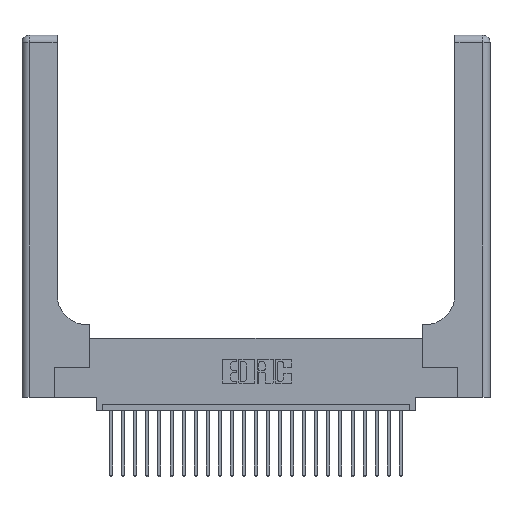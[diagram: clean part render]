
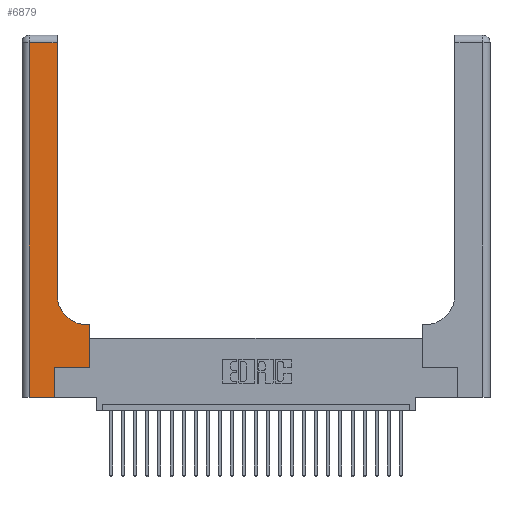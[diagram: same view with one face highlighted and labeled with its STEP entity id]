
A CAD part, top view. The second image highlights one B-rep face of the part: STEP entity #6879.
In plain terms, the highlighted planar face has unit normal (0, 0, 1).
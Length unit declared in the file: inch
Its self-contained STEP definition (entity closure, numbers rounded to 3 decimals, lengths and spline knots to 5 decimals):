
#257 = CARTESIAN_POINT ( 'NONE',  ( 0.2915, 0.6, 0.37 ) ) ;
#272 = VECTOR ( 'NONE', #532, 39.37008 ) ;
#532 = DIRECTION ( 'NONE',  ( -1., 0., 0. ) ) ;
#700 = VECTOR ( 'NONE', #7578, 39.37008 ) ;
#1446 = EDGE_CURVE ( 'NONE', #2552, #12616, #8903, .T. ) ;
#1455 = ORIENTED_EDGE ( 'NONE', *, *, #1446, .T. ) ;
#2546 = VECTOR ( 'NONE', #20763, 39.37008 ) ;
#2552 = VERTEX_POINT ( 'NONE', #17194 ) ;
#2687 = EDGE_CURVE ( 'NONE', #10802, #5276, #7561, .T. ) ;
#2690 = ORIENTED_EDGE ( 'NONE', *, *, #9593, .T. ) ;
#3460 = DIRECTION ( 'NONE',  ( 0., 1., 0. ) ) ;
#3850 = CARTESIAN_POINT ( 'NONE',  ( 0.269, 0., 0.37 ) ) ;
#4066 = DIRECTION ( 'NONE',  ( -1., 0., 0. ) ) ;
#4154 = EDGE_CURVE ( 'NONE', #20990, #23542, #19220, .T. ) ;
#4846 = ORIENTED_EDGE ( 'NONE', *, *, #2687, .T. ) ;
#5008 = CARTESIAN_POINT ( 'NONE',  ( 0.269, 0.25, 0.37 ) ) ;
#5019 = CARTESIAN_POINT ( 'NONE',  ( 0.2915, 2.94, 0.37 ) ) ;
#5276 = VERTEX_POINT ( 'NONE', #5019 ) ;
#5653 = ORIENTED_EDGE ( 'NONE', *, *, #4154, .T. ) ;
#6140 = CARTESIAN_POINT ( 'NONE',  ( 0.269, 0., 0.37 ) ) ;
#6418 = LINE ( 'NONE', #3850, #23957 ) ;
#6633 = VECTOR ( 'NONE', #10738, 39.37008 ) ;
#6695 = CARTESIAN_POINT ( 'NONE',  ( 0.06, 3., 0.37 ) ) ;
#6803 = ORIENTED_EDGE ( 'NONE', *, *, #17563, .T. ) ;
#6879 = ADVANCED_FACE ( 'NONE', ( #11767 ), #23981, .F. ) ;
#7432 = EDGE_CURVE ( 'NONE', #16735, #2552, #18145, .T. ) ;
#7561 = LINE ( 'NONE', #25804, #24455 ) ;
#7578 = DIRECTION ( 'NONE',  ( 1., 0., 0. ) ) ;
#8582 = VERTEX_POINT ( 'NONE', #22596 ) ;
#8672 = DIRECTION ( 'NONE',  ( 1., 0., 0. ) ) ;
#8835 = CARTESIAN_POINT ( 'NONE',  ( 0., 2.94, 0.37 ) ) ;
#8903 = LINE ( 'NONE', #257, #272 ) ;
#9299 = EDGE_LOOP ( 'NONE', ( #4846, #2690, #24433, #5653, #21065, #9450, #14079, #1455, #6803 ) ) ;
#9450 = ORIENTED_EDGE ( 'NONE', *, *, #22508, .T. ) ;
#9593 = EDGE_CURVE ( 'NONE', #5276, #20825, #26169, .T. ) ;
#10149 = AXIS2_PLACEMENT_3D ( 'NONE', #19183, #21195, #8672 ) ;
#10492 = CARTESIAN_POINT ( 'NONE',  ( 0.5585, 0.25, 0.37 ) ) ;
#10738 = DIRECTION ( 'NONE',  ( 0., -1., 0. ) ) ;
#10802 = VERTEX_POINT ( 'NONE', #23255 ) ;
#11433 = LINE ( 'NONE', #5008, #24173 ) ;
#11767 = FACE_OUTER_BOUND ( 'NONE', #9299, .T. ) ;
#12616 = VERTEX_POINT ( 'NONE', #16531 ) ;
#12653 = AXIS2_PLACEMENT_3D ( 'NONE', #23078, #13308, #4066 ) ;
#12728 = CIRCLE ( 'NONE', #10149, 0.25 ) ;
#13308 = DIRECTION ( 'NONE',  ( 0., 0., -1. ) ) ;
#14079 = ORIENTED_EDGE ( 'NONE', *, *, #7432, .T. ) ;
#15754 = CARTESIAN_POINT ( 'NONE',  ( 0.06, 0., 0.37 ) ) ;
#16531 = CARTESIAN_POINT ( 'NONE',  ( 0.5415, 0.6, 0.37 ) ) ;
#16735 = VERTEX_POINT ( 'NONE', #10492 ) ;
#17194 = CARTESIAN_POINT ( 'NONE',  ( 0.5585, 0.6, 0.37 ) ) ;
#17563 = EDGE_CURVE ( 'NONE', #12616, #10802, #12728, .T. ) ;
#17808 = VECTOR ( 'NONE', #20792, 39.37008 ) ;
#18145 = LINE ( 'NONE', #18601, #17808 ) ;
#18601 = CARTESIAN_POINT ( 'NONE',  ( 0.5585, 0.25, 0.37 ) ) ;
#19183 = CARTESIAN_POINT ( 'NONE',  ( 0.5415, 0.85, 0.37 ) ) ;
#19220 = LINE ( 'NONE', #19799, #700 ) ;
#19799 = CARTESIAN_POINT ( 'NONE',  ( 0., 0., 0.37 ) ) ;
#20053 = LINE ( 'NONE', #6695, #6633 ) ;
#20763 = DIRECTION ( 'NONE',  ( -1., 0., 0. ) ) ;
#20792 = DIRECTION ( 'NONE',  ( 0., 1., 0. ) ) ;
#20825 = VERTEX_POINT ( 'NONE', #24700 ) ;
#20990 = VERTEX_POINT ( 'NONE', #15754 ) ;
#21065 = ORIENTED_EDGE ( 'NONE', *, *, #21072, .T. ) ;
#21072 = EDGE_CURVE ( 'NONE', #23542, #8582, #6418, .T. ) ;
#21195 = DIRECTION ( 'NONE',  ( 0., 0., -1. ) ) ;
#22508 = EDGE_CURVE ( 'NONE', #8582, #16735, #11433, .T. ) ;
#22596 = CARTESIAN_POINT ( 'NONE',  ( 0.269, 0.25, 0.37 ) ) ;
#22633 = EDGE_CURVE ( 'NONE', #20825, #20990, #20053, .T. ) ;
#23078 = CARTESIAN_POINT ( 'NONE',  ( 0., 3., 0.37 ) ) ;
#23255 = CARTESIAN_POINT ( 'NONE',  ( 0.2915, 0.85, 0.37 ) ) ;
#23542 = VERTEX_POINT ( 'NONE', #6140 ) ;
#23957 = VECTOR ( 'NONE', #26027, 39.37008 ) ;
#23981 = PLANE ( 'NONE',  #12653 ) ;
#24173 = VECTOR ( 'NONE', #25143, 39.37008 ) ;
#24433 = ORIENTED_EDGE ( 'NONE', *, *, #22633, .T. ) ;
#24455 = VECTOR ( 'NONE', #3460, 39.37008 ) ;
#24700 = CARTESIAN_POINT ( 'NONE',  ( 0.06, 2.94, 0.37 ) ) ;
#25143 = DIRECTION ( 'NONE',  ( 1., 0., 0. ) ) ;
#25804 = CARTESIAN_POINT ( 'NONE',  ( 0.2915, 3., 0.37 ) ) ;
#26027 = DIRECTION ( 'NONE',  ( 0., 1., 0. ) ) ;
#26169 = LINE ( 'NONE', #8835, #2546 ) ;
